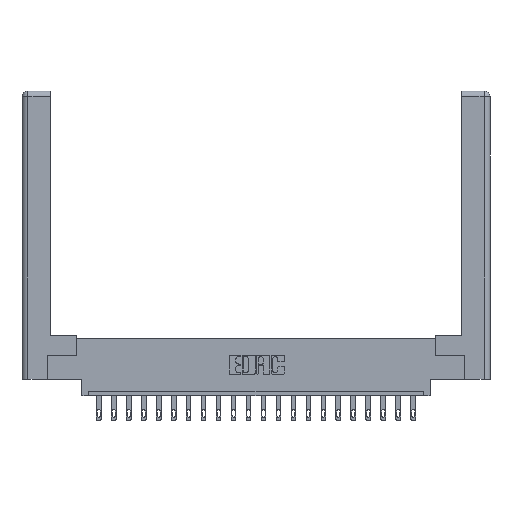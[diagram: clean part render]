
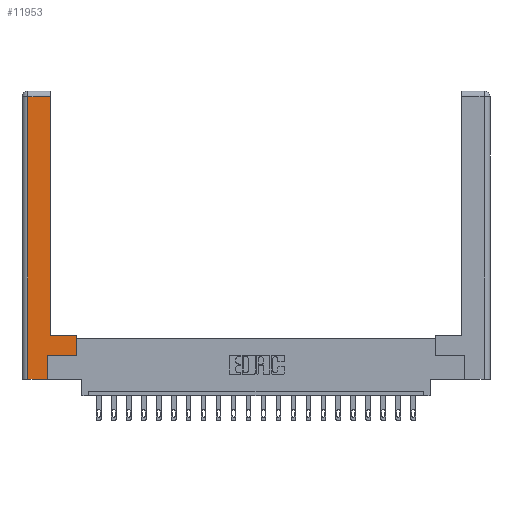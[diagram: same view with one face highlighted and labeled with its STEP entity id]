
A CAD part, top view. The second image highlights one B-rep face of the part: STEP entity #11953.
In plain terms, the highlighted planar face has unit normal (0, 0, 1).
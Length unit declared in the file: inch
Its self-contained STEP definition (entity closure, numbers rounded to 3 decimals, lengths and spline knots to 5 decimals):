
#32 = ORIENTED_EDGE ( 'NONE', *, *, #7172, .T. ) ;
#65 = EDGE_CURVE ( 'NONE', #2369, #6950, #5176, .T. ) ;
#928 = VERTEX_POINT ( 'NONE', #19713 ) ;
#962 = CARTESIAN_POINT ( 'NONE',  ( 0., 0., 0. ) ) ;
#1070 = LINE ( 'NONE', #11048, #11120 ) ;
#1672 = CARTESIAN_POINT ( 'NONE',  ( 0.0615, 2.94, 0. ) ) ;
#2332 = VERTEX_POINT ( 'NONE', #20830 ) ;
#2369 = VERTEX_POINT ( 'NONE', #17413 ) ;
#2658 = DIRECTION ( 'NONE',  ( -1., 0., 0. ) ) ;
#3590 = EDGE_CURVE ( 'NONE', #928, #12491, #20938, .T. ) ;
#4349 = VECTOR ( 'NONE', #21556, 39.37008 ) ;
#4431 = LINE ( 'NONE', #7447, #19350 ) ;
#4457 = DIRECTION ( 'NONE',  ( 1., 0., 0. ) ) ;
#4634 = VECTOR ( 'NONE', #4457, 39.37008 ) ;
#4716 = VECTOR ( 'NONE', #2658, 39.37008 ) ;
#4826 = EDGE_LOOP ( 'NONE', ( #6602, #9270, #5541, #6865, #19285, #20691, #14308, #32 ) ) ;
#5176 = LINE ( 'NONE', #6001, #4634 ) ;
#5541 = ORIENTED_EDGE ( 'NONE', *, *, #14106, .T. ) ;
#5783 = CARTESIAN_POINT ( 'NONE',  ( 0.265, 0., 0. ) ) ;
#5886 = CARTESIAN_POINT ( 'NONE',  ( 0.0615, 2.94, 0. ) ) ;
#6001 = CARTESIAN_POINT ( 'NONE',  ( 0.265, 0., 0. ) ) ;
#6228 = DIRECTION ( 'NONE',  ( 0., 0., -1. ) ) ;
#6401 = EDGE_CURVE ( 'NONE', #15087, #2332, #9654, .T. ) ;
#6602 = ORIENTED_EDGE ( 'NONE', *, *, #14481, .T. ) ;
#6865 = ORIENTED_EDGE ( 'NONE', *, *, #65, .T. ) ;
#6950 = VERTEX_POINT ( 'NONE', #5783 ) ;
#7172 = EDGE_CURVE ( 'NONE', #13919, #21059, #21097, .T. ) ;
#7447 = CARTESIAN_POINT ( 'NONE',  ( 0.0615, 0., 0. ) ) ;
#7620 = DIRECTION ( 'NONE',  ( -1., 0., 0. ) ) ;
#8108 = CARTESIAN_POINT ( 'NONE',  ( 0.295, 0.45, 0. ) ) ;
#8554 = CARTESIAN_POINT ( 'NONE',  ( 0.265, 0.245, 0. ) ) ;
#9270 = ORIENTED_EDGE ( 'NONE', *, *, #3590, .T. ) ;
#9309 = DIRECTION ( 'NONE',  ( 0., 1., 0. ) ) ;
#9654 = LINE ( 'NONE', #16364, #10979 ) ;
#10201 = FACE_OUTER_BOUND ( 'NONE', #4826, .T. ) ;
#10359 = CARTESIAN_POINT ( 'NONE',  ( 0.565, 0.45, 0. ) ) ;
#10716 = DIRECTION ( 'NONE',  ( 0., -1., 0. ) ) ;
#10979 = VECTOR ( 'NONE', #17902, 39.37008 ) ;
#11048 = CARTESIAN_POINT ( 'NONE',  ( 0.565, 0.45, 0. ) ) ;
#11112 = AXIS2_PLACEMENT_3D ( 'NONE', #962, #6228, #7620 ) ;
#11120 = VECTOR ( 'NONE', #21101, 39.37008 ) ;
#11232 = PLANE ( 'NONE',  #11112 ) ;
#11260 = VECTOR ( 'NONE', #9309, 39.37008 ) ;
#11953 = ADVANCED_FACE ( 'NONE', ( #10201 ), #11232, .F. ) ;
#12201 = EDGE_CURVE ( 'NONE', #6950, #15087, #15002, .T. ) ;
#12491 = VERTEX_POINT ( 'NONE', #1672 ) ;
#12842 = CARTESIAN_POINT ( 'NONE',  ( 0.295, 3., 0. ) ) ;
#12902 = VECTOR ( 'NONE', #15596, 39.37008 ) ;
#13919 = VERTEX_POINT ( 'NONE', #10359 ) ;
#14106 = EDGE_CURVE ( 'NONE', #12491, #2369, #4431, .T. ) ;
#14308 = ORIENTED_EDGE ( 'NONE', *, *, #18007, .T. ) ;
#14481 = EDGE_CURVE ( 'NONE', #21059, #928, #16479, .T. ) ;
#15002 = LINE ( 'NONE', #18885, #12902 ) ;
#15087 = VERTEX_POINT ( 'NONE', #8554 ) ;
#15596 = DIRECTION ( 'NONE',  ( 0., 1., 0. ) ) ;
#16364 = CARTESIAN_POINT ( 'NONE',  ( 0.565, 0.245, 0. ) ) ;
#16479 = LINE ( 'NONE', #12842, #11260 ) ;
#16532 = CARTESIAN_POINT ( 'NONE',  ( 0.295, 0.45, 0. ) ) ;
#17413 = CARTESIAN_POINT ( 'NONE',  ( 0.0615, 0., 0. ) ) ;
#17902 = DIRECTION ( 'NONE',  ( 1., 0., 0. ) ) ;
#18007 = EDGE_CURVE ( 'NONE', #2332, #13919, #1070, .T. ) ;
#18885 = CARTESIAN_POINT ( 'NONE',  ( 0.265, 0.245, 0. ) ) ;
#19285 = ORIENTED_EDGE ( 'NONE', *, *, #12201, .T. ) ;
#19350 = VECTOR ( 'NONE', #10716, 39.37008 ) ;
#19713 = CARTESIAN_POINT ( 'NONE',  ( 0.295, 2.94, 0. ) ) ;
#20691 = ORIENTED_EDGE ( 'NONE', *, *, #6401, .T. ) ;
#20830 = CARTESIAN_POINT ( 'NONE',  ( 0.565, 0.245, 0. ) ) ;
#20938 = LINE ( 'NONE', #5886, #4716 ) ;
#21059 = VERTEX_POINT ( 'NONE', #8108 ) ;
#21097 = LINE ( 'NONE', #16532, #4349 ) ;
#21101 = DIRECTION ( 'NONE',  ( 0., 1., 0. ) ) ;
#21556 = DIRECTION ( 'NONE',  ( -1., 0., 0. ) ) ;
